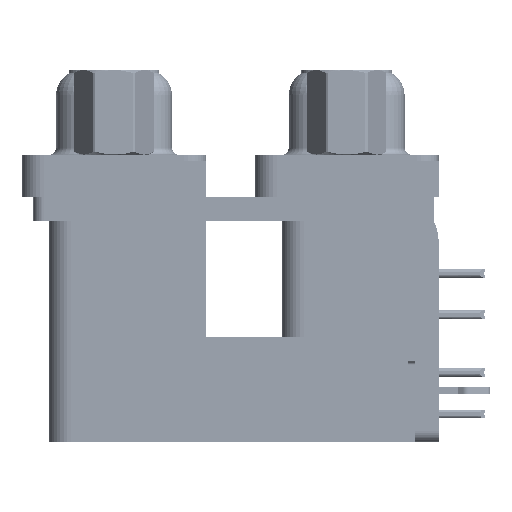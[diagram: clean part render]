
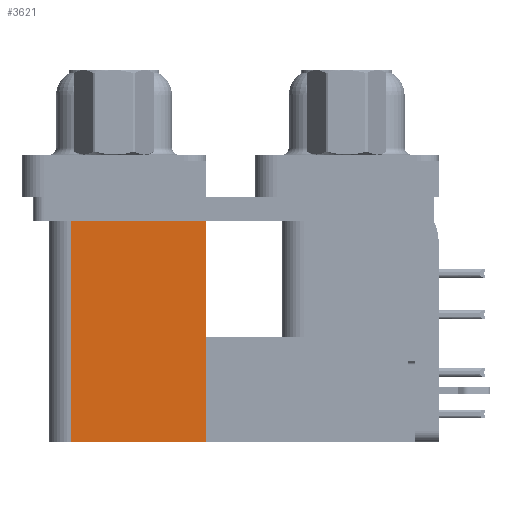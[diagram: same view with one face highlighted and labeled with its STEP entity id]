
A CAD part, left-side view. The second image highlights one B-rep face of the part: STEP entity #3621.
In plain terms, the highlighted planar face has unit normal (-1, 0, 0).
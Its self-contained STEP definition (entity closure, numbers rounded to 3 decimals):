
#299 = CARTESIAN_POINT ( 'NONE',  ( 3.7, 9.6, -19.2 ) ) ;
#1800 = ORIENTED_EDGE ( 'NONE', *, *, #55658, .F. ) ;
#2644 = DIRECTION ( 'NONE',  ( 0., 1., 0. ) ) ;
#2660 = DIRECTION ( 'NONE',  ( 0., 1., 0. ) ) ;
#3567 = AXIS2_PLACEMENT_3D ( 'NONE', #61163, #60566, #18809 ) ;
#3621 = ADVANCED_FACE ( 'NONE', ( #19719 ), #40472, .F. ) ;
#4009 = DIRECTION ( 'NONE',  ( 0., 0., 1. ) ) ;
#5024 = EDGE_LOOP ( 'NONE', ( #50963, #1800, #51124, #5126 ) ) ;
#5126 = ORIENTED_EDGE ( 'NONE', *, *, #56002, .T. ) ;
#5418 = EDGE_CURVE ( 'NONE', #57027, #49838, #7420, .T. ) ;
#7420 = LINE ( 'NONE', #48241, #66531 ) ;
#7716 = VECTOR ( 'NONE', #4009, 1000. ) ;
#11424 = CARTESIAN_POINT ( 'NONE',  ( 3.7, 18.8, -2.5 ) ) ;
#15039 = VECTOR ( 'NONE', #2644, 1000. ) ;
#18809 = DIRECTION ( 'NONE',  ( 0., 1., 0. ) ) ;
#19719 = FACE_OUTER_BOUND ( 'NONE', #5024, .T. ) ;
#23046 = CARTESIAN_POINT ( 'NONE',  ( 3.7, 9.6, -2.5 ) ) ;
#29885 = CARTESIAN_POINT ( 'NONE',  ( 3.7, 9.6, -19.2 ) ) ;
#31292 = CARTESIAN_POINT ( 'NONE',  ( 3.7, 9.6, -2.5 ) ) ;
#31686 = VECTOR ( 'NONE', #52587, 1000. ) ;
#34548 = VERTEX_POINT ( 'NONE', #11424 ) ;
#38523 = CARTESIAN_POINT ( 'NONE',  ( 3.7, 18.8, -19.2 ) ) ;
#39253 = EDGE_CURVE ( 'NONE', #46565, #34548, #59067, .T. ) ;
#40472 = PLANE ( 'NONE',  #3567 ) ;
#42405 = LINE ( 'NONE', #42737, #31686 ) ;
#42737 = CARTESIAN_POINT ( 'NONE',  ( 3.7, 18.8, -19.2 ) ) ;
#46565 = VERTEX_POINT ( 'NONE', #31292 ) ;
#48241 = CARTESIAN_POINT ( 'NONE',  ( 3.7, 9.6, -19.2 ) ) ;
#49838 = VERTEX_POINT ( 'NONE', #38523 ) ;
#50963 = ORIENTED_EDGE ( 'NONE', *, *, #39253, .T. ) ;
#51124 = ORIENTED_EDGE ( 'NONE', *, *, #5418, .F. ) ;
#52587 = DIRECTION ( 'NONE',  ( 0., 0., 1. ) ) ;
#55658 = EDGE_CURVE ( 'NONE', #49838, #34548, #42405, .T. ) ;
#56002 = EDGE_CURVE ( 'NONE', #57027, #46565, #61122, .T. ) ;
#57027 = VERTEX_POINT ( 'NONE', #29885 ) ;
#59067 = LINE ( 'NONE', #23046, #15039 ) ;
#60566 = DIRECTION ( 'NONE',  ( 1., 0., 0. ) ) ;
#61122 = LINE ( 'NONE', #299, #7716 ) ;
#61163 = CARTESIAN_POINT ( 'NONE',  ( 3.7, 9.6, -19.2 ) ) ;
#66531 = VECTOR ( 'NONE', #2660, 1000. ) ;
